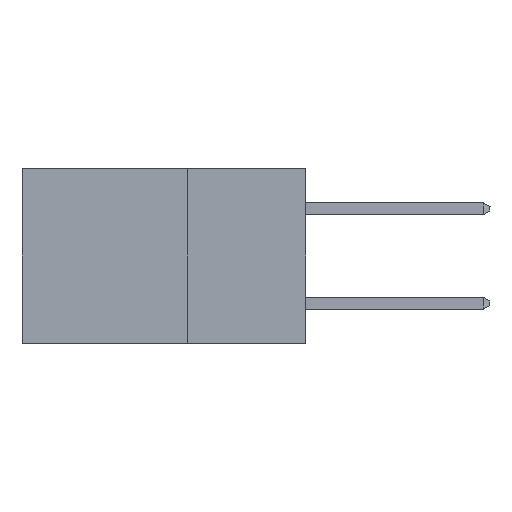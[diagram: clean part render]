
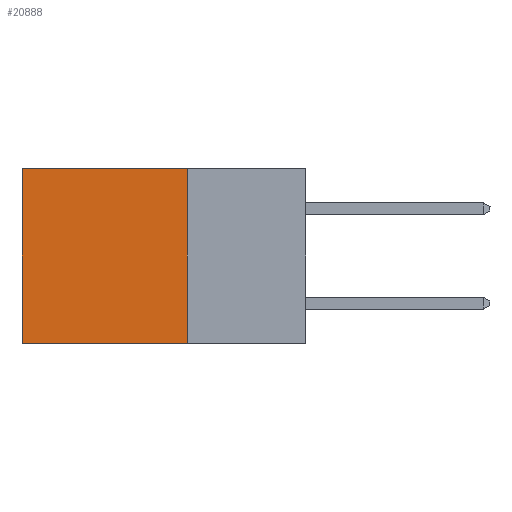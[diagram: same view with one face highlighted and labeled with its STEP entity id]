
A CAD part, left-side view. The second image highlights one B-rep face of the part: STEP entity #20888.
In plain terms, the highlighted planar face has unit normal (-1, 0, 0).
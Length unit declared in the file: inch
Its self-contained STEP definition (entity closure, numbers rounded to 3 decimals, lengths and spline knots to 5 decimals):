
#1352 = CARTESIAN_POINT ( 'NONE',  ( 0.298, 0.6, -0.37 ) ) ;
#2884 = CARTESIAN_POINT ( 'NONE',  ( 0.298, 0.25, 0. ) ) ;
#3755 = EDGE_CURVE ( 'NONE', #11918, #27702, #21075, .T. ) ;
#3965 = ORIENTED_EDGE ( 'NONE', *, *, #25225, .T. ) ;
#4171 = VECTOR ( 'NONE', #24112, 39.37008 ) ;
#4534 = CARTESIAN_POINT ( 'NONE',  ( 0.298, 0.6, 0. ) ) ;
#5348 = DIRECTION ( 'NONE',  ( 0., 0., -1. ) ) ;
#6538 = CARTESIAN_POINT ( 'NONE',  ( 0.298, 0.25, -0.37 ) ) ;
#7282 = ORIENTED_EDGE ( 'NONE', *, *, #3755, .F. ) ;
#9950 = FACE_OUTER_BOUND ( 'NONE', #13613, .T. ) ;
#11918 = VERTEX_POINT ( 'NONE', #6538 ) ;
#12578 = PLANE ( 'NONE',  #24403 ) ;
#12984 = ORIENTED_EDGE ( 'NONE', *, *, #28678, .F. ) ;
#13613 = EDGE_LOOP ( 'NONE', ( #14970, #7282, #12984, #3965 ) ) ;
#13930 = VECTOR ( 'NONE', #29836, 39.37008 ) ;
#14434 = CARTESIAN_POINT ( 'NONE',  ( 0.298, 0.25, 0. ) ) ;
#14970 = ORIENTED_EDGE ( 'NONE', *, *, #22201, .T. ) ;
#15965 = VECTOR ( 'NONE', #16207, 39.37008 ) ;
#16207 = DIRECTION ( 'NONE',  ( 0., 1., 0. ) ) ;
#16877 = DIRECTION ( 'NONE',  ( 0., 0., -1. ) ) ;
#17023 = CARTESIAN_POINT ( 'NONE',  ( 0.298, 0.6, 0. ) ) ;
#17042 = LINE ( 'NONE', #17023, #4171 ) ;
#18451 = VERTEX_POINT ( 'NONE', #4534 ) ;
#19581 = LINE ( 'NONE', #14434, #25199 ) ;
#19805 = DIRECTION ( 'NONE',  ( 1., 0., 0. ) ) ;
#20888 = ADVANCED_FACE ( 'NONE', ( #9950 ), #12578, .F. ) ;
#21075 = LINE ( 'NONE', #21657, #13930 ) ;
#21657 = CARTESIAN_POINT ( 'NONE',  ( 0.298, 0.25, -0.37 ) ) ;
#22025 = CARTESIAN_POINT ( 'NONE',  ( 0.298, 0.25, 0. ) ) ;
#22201 = EDGE_CURVE ( 'NONE', #18451, #27702, #17042, .T. ) ;
#24112 = DIRECTION ( 'NONE',  ( 0., 0., -1. ) ) ;
#24403 = AXIS2_PLACEMENT_3D ( 'NONE', #2884, #19805, #5348 ) ;
#25199 = VECTOR ( 'NONE', #16877, 39.37008 ) ;
#25225 = EDGE_CURVE ( 'NONE', #28070, #18451, #28695, .T. ) ;
#27702 = VERTEX_POINT ( 'NONE', #1352 ) ;
#28070 = VERTEX_POINT ( 'NONE', #22025 ) ;
#28678 = EDGE_CURVE ( 'NONE', #28070, #11918, #19581, .T. ) ;
#28695 = LINE ( 'NONE', #30405, #15965 ) ;
#29836 = DIRECTION ( 'NONE',  ( 0., 1., 0. ) ) ;
#30405 = CARTESIAN_POINT ( 'NONE',  ( 0.298, 0.25, 0. ) ) ;
